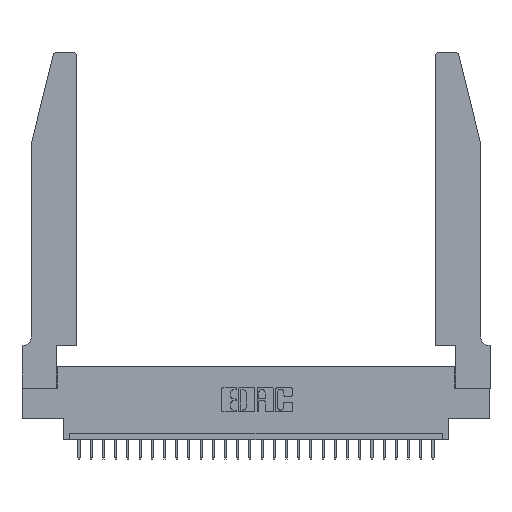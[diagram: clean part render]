
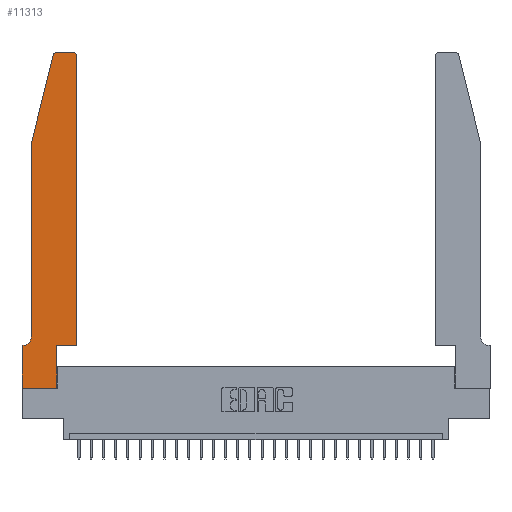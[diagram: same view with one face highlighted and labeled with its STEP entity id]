
A CAD part, top view. The second image highlights one B-rep face of the part: STEP entity #11313.
In plain terms, the highlighted planar face has unit normal (0, 0, 1).
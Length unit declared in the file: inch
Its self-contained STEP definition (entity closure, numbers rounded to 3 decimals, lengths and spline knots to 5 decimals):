
#400 = VERTEX_POINT ( 'NONE', #16940 ) ;
#848 = VECTOR ( 'NONE', #24264, 39.37008 ) ;
#889 = ORIENTED_EDGE ( 'NONE', *, *, #27318, .T. ) ;
#1440 = CARTESIAN_POINT ( 'NONE',  ( 0.4505, 2.72, 0.37 ) ) ;
#1710 = DIRECTION ( 'NONE',  ( 1., 0., 0. ) ) ;
#1982 = VERTEX_POINT ( 'NONE', #22952 ) ;
#2248 = EDGE_CURVE ( 'NONE', #20824, #400, #27184, .T. ) ;
#3127 = LINE ( 'NONE', #27288, #20675 ) ;
#3434 = ORIENTED_EDGE ( 'NONE', *, *, #21252, .T. ) ;
#5019 = VECTOR ( 'NONE', #16967, 39.37008 ) ;
#5253 = CARTESIAN_POINT ( 'NONE',  ( 0.284, 2.75, 0.37 ) ) ;
#5301 = EDGE_CURVE ( 'NONE', #19730, #16291, #22889, .T. ) ;
#6122 = DIRECTION ( 'NONE',  ( 0., 0., -1. ) ) ;
#6175 = CARTESIAN_POINT ( 'NONE',  ( 0.0755, 2., 0.37 ) ) ;
#6270 = CARTESIAN_POINT ( 'NONE',  ( 0.4205, 2.75, 0.37 ) ) ;
#6322 = DIRECTION ( 'NONE',  ( 1., 0., 0. ) ) ;
#6345 = ORIENTED_EDGE ( 'NONE', *, *, #5301, .T. ) ;
#6516 = DIRECTION ( 'NONE',  ( -1., 0., 0. ) ) ;
#6718 = DIRECTION ( 'NONE',  ( 1., 0., 0. ) ) ;
#6866 = VERTEX_POINT ( 'NONE', #13799 ) ;
#7856 = EDGE_CURVE ( 'NONE', #400, #27487, #18562, .T. ) ;
#7973 = DIRECTION ( 'NONE',  ( -1., 0., 0. ) ) ;
#8097 = ORIENTED_EDGE ( 'NONE', *, *, #7856, .T. ) ;
#8168 = AXIS2_PLACEMENT_3D ( 'NONE', #26503, #24307, #6718 ) ;
#9200 = VERTEX_POINT ( 'NONE', #14788 ) ;
#9206 = DIRECTION ( 'NONE',  ( 0., 1., 0. ) ) ;
#9382 = ORIENTED_EDGE ( 'NONE', *, *, #18788, .T. ) ;
#9403 = CIRCLE ( 'NONE', #8168, 0.03 ) ;
#10330 = VERTEX_POINT ( 'NONE', #25801 ) ;
#10604 = AXIS2_PLACEMENT_3D ( 'NONE', #17203, #28653, #1710 ) ;
#10742 = CARTESIAN_POINT ( 'NONE',  ( 0.0755, 2., 0.37 ) ) ;
#11313 = ADVANCED_FACE ( 'NONE', ( #17112 ), #22104, .T. ) ;
#11373 = LINE ( 'NONE', #10742, #5019 ) ;
#11453 = CARTESIAN_POINT ( 'NONE',  ( 0.2865, 0.35, 0.37 ) ) ;
#12708 = EDGE_CURVE ( 'NONE', #16291, #1982, #27954, .T. ) ;
#13003 = CARTESIAN_POINT ( 'NONE',  ( 0.4505, 0.35, 0.37 ) ) ;
#13799 = CARTESIAN_POINT ( 'NONE',  ( 0.0055, 0.35, 0.37 ) ) ;
#13942 = EDGE_CURVE ( 'NONE', #19612, #10330, #11373, .T. ) ;
#14439 = EDGE_CURVE ( 'NONE', #15657, #20824, #25376, .T. ) ;
#14788 = CARTESIAN_POINT ( 'NONE',  ( 0., 0.35, 0.37 ) ) ;
#15216 = VECTOR ( 'NONE', #17491, 39.37008 ) ;
#15292 = LINE ( 'NONE', #20466, #848 ) ;
#15531 = VECTOR ( 'NONE', #9206, 39.37008 ) ;
#15534 = VECTOR ( 'NONE', #18979, 39.37008 ) ;
#15613 = EDGE_CURVE ( 'NONE', #10330, #6866, #16542, .T. ) ;
#15649 = VECTOR ( 'NONE', #27012, 39.37008 ) ;
#15657 = VERTEX_POINT ( 'NONE', #20243 ) ;
#16188 = ORIENTED_EDGE ( 'NONE', *, *, #23294, .T. ) ;
#16291 = VERTEX_POINT ( 'NONE', #5253 ) ;
#16325 = LINE ( 'NONE', #24738, #15649 ) ;
#16542 = CIRCLE ( 'NONE', #28389, 0.07 ) ;
#16940 = CARTESIAN_POINT ( 'NONE',  ( 0.4505, 0.35, 0.37 ) ) ;
#16967 = DIRECTION ( 'NONE',  ( 0., -1., 0. ) ) ;
#17112 = FACE_OUTER_BOUND ( 'NONE', #23313, .T. ) ;
#17203 = CARTESIAN_POINT ( 'NONE',  ( 0.284, 2.72, 0.37 ) ) ;
#17491 = DIRECTION ( 'NONE',  ( 1., 0., 0. ) ) ;
#17911 = AXIS2_PLACEMENT_3D ( 'NONE', #26765, #19754, #6322 ) ;
#18562 = LINE ( 'NONE', #19489, #23138 ) ;
#18788 = EDGE_CURVE ( 'NONE', #6866, #9200, #28632, .T. ) ;
#18979 = DIRECTION ( 'NONE',  ( -1., 0., 0. ) ) ;
#19083 = CARTESIAN_POINT ( 'NONE',  ( 0.2605, 2.75, 0.37 ) ) ;
#19387 = VERTEX_POINT ( 'NONE', #27006 ) ;
#19489 = CARTESIAN_POINT ( 'NONE',  ( 0.4505, 0.35, 0.37 ) ) ;
#19534 = CARTESIAN_POINT ( 'NONE',  ( 0.0055, 0.42, 0.37 ) ) ;
#19612 = VERTEX_POINT ( 'NONE', #6175 ) ;
#19623 = ORIENTED_EDGE ( 'NONE', *, *, #13942, .T. ) ;
#19730 = VERTEX_POINT ( 'NONE', #6270 ) ;
#19752 = CARTESIAN_POINT ( 'NONE',  ( 0.0755, 0.35, 0.37 ) ) ;
#19754 = DIRECTION ( 'NONE',  ( 0., 0., 1. ) ) ;
#19757 = ORIENTED_EDGE ( 'NONE', *, *, #24001, .T. ) ;
#20243 = CARTESIAN_POINT ( 'NONE',  ( 0.2865, 0., 0.37 ) ) ;
#20466 = CARTESIAN_POINT ( 'NONE',  ( 0., 0., 0.37 ) ) ;
#20471 = DIRECTION ( 'NONE',  ( -0.239, -0.971, 0. ) ) ;
#20675 = VECTOR ( 'NONE', #20471, 39.37008 ) ;
#20824 = VERTEX_POINT ( 'NONE', #25236 ) ;
#20830 = VECTOR ( 'NONE', #6516, 39.37008 ) ;
#21252 = EDGE_CURVE ( 'NONE', #9200, #19387, #15292, .T. ) ;
#22104 = PLANE ( 'NONE',  #17911 ) ;
#22889 = LINE ( 'NONE', #19083, #15534 ) ;
#22952 = CARTESIAN_POINT ( 'NONE',  ( 0.25487, 2.72718, 0.37 ) ) ;
#23138 = VECTOR ( 'NONE', #23727, 39.37008 ) ;
#23294 = EDGE_CURVE ( 'NONE', #27487, #19730, #9403, .T. ) ;
#23313 = EDGE_LOOP ( 'NONE', ( #6345, #27273, #889, #19623, #26673, #9382, #3434, #19757, #27429, #25525, #8097, #16188 ) ) ;
#23727 = DIRECTION ( 'NONE',  ( 0., 1., 0. ) ) ;
#24001 = EDGE_CURVE ( 'NONE', #19387, #15657, #16325, .T. ) ;
#24264 = DIRECTION ( 'NONE',  ( 0., -1., 0. ) ) ;
#24307 = DIRECTION ( 'NONE',  ( 0., 0., 1. ) ) ;
#24738 = CARTESIAN_POINT ( 'NONE',  ( 0., 0., 0.37 ) ) ;
#25236 = CARTESIAN_POINT ( 'NONE',  ( 0.2865, 0.35, 0.37 ) ) ;
#25376 = LINE ( 'NONE', #11453, #15531 ) ;
#25525 = ORIENTED_EDGE ( 'NONE', *, *, #2248, .T. ) ;
#25801 = CARTESIAN_POINT ( 'NONE',  ( 0.0755, 0.42, 0.37 ) ) ;
#26503 = CARTESIAN_POINT ( 'NONE',  ( 0.4205, 2.72, 0.37 ) ) ;
#26673 = ORIENTED_EDGE ( 'NONE', *, *, #15613, .T. ) ;
#26765 = CARTESIAN_POINT ( 'NONE',  ( 0., 0.35, 0.37 ) ) ;
#27006 = CARTESIAN_POINT ( 'NONE',  ( 0., 0., 0.37 ) ) ;
#27012 = DIRECTION ( 'NONE',  ( 1., 0., 0. ) ) ;
#27184 = LINE ( 'NONE', #13003, #15216 ) ;
#27273 = ORIENTED_EDGE ( 'NONE', *, *, #12708, .T. ) ;
#27288 = CARTESIAN_POINT ( 'NONE',  ( 0.0755, 2., 0.37 ) ) ;
#27318 = EDGE_CURVE ( 'NONE', #1982, #19612, #3127, .T. ) ;
#27429 = ORIENTED_EDGE ( 'NONE', *, *, #14439, .T. ) ;
#27487 = VERTEX_POINT ( 'NONE', #1440 ) ;
#27954 = CIRCLE ( 'NONE', #10604, 0.03 ) ;
#28389 = AXIS2_PLACEMENT_3D ( 'NONE', #19534, #6122, #7973 ) ;
#28632 = LINE ( 'NONE', #19752, #20830 ) ;
#28653 = DIRECTION ( 'NONE',  ( 0., 0., 1. ) ) ;
